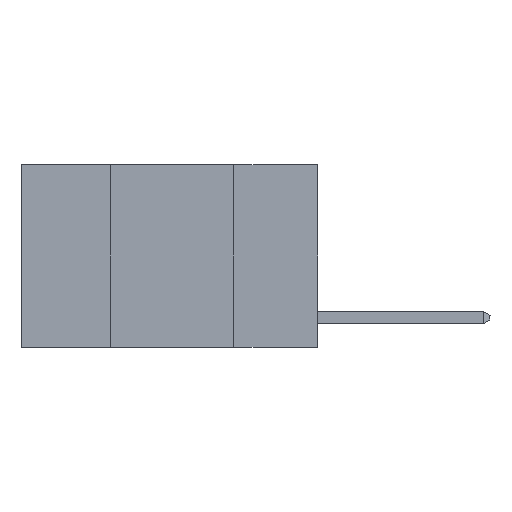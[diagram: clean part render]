
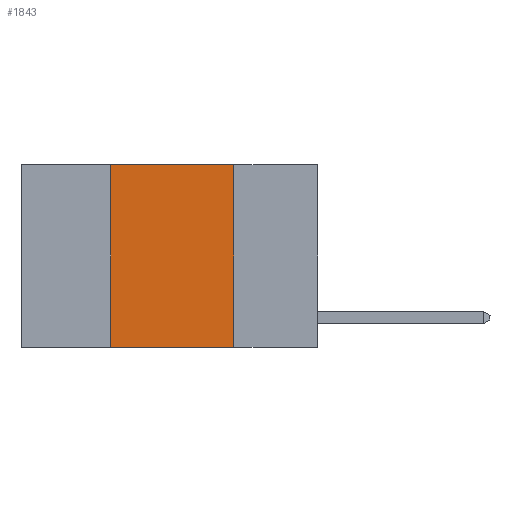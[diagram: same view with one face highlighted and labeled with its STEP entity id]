
A CAD part, left-side view. The second image highlights one B-rep face of the part: STEP entity #1843.
In plain terms, the highlighted planar face has unit normal (-1, 0, 0).
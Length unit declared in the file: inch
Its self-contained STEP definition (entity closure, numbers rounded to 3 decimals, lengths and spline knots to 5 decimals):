
#255 = EDGE_CURVE ( 'NONE', #11716, #3188, #11591, .T. ) ;
#520 = DIRECTION ( 'NONE',  ( 0., 0., -1. ) ) ;
#623 = LINE ( 'NONE', #10153, #10955 ) ;
#773 = EDGE_CURVE ( 'NONE', #4697, #6847, #623, .T. ) ;
#774 = AXIS2_PLACEMENT_3D ( 'NONE', #5759, #6787, #520 ) ;
#1813 = ORIENTED_EDGE ( 'NONE', *, *, #255, .T. ) ;
#1843 = ADVANCED_FACE ( 'NONE', ( #6644 ), #11828, .F. ) ;
#1957 = CARTESIAN_POINT ( 'NONE',  ( 0., 0.42, -0.37 ) ) ;
#2440 = ORIENTED_EDGE ( 'NONE', *, *, #3088, .F. ) ;
#2998 = DIRECTION ( 'NONE',  ( 0., -1., 0. ) ) ;
#3088 = EDGE_CURVE ( 'NONE', #11716, #4697, #7552, .T. ) ;
#3188 = VERTEX_POINT ( 'NONE', #8435 ) ;
#3421 = VECTOR ( 'NONE', #2998, 39.37008 ) ;
#3844 = CARTESIAN_POINT ( 'NONE',  ( 0., 0.42, 0. ) ) ;
#4002 = DIRECTION ( 'NONE',  ( 0., -1., 0. ) ) ;
#4008 = EDGE_LOOP ( 'NONE', ( #4565, #5241, #2440, #1813 ) ) ;
#4195 = VECTOR ( 'NONE', #5495, 39.37008 ) ;
#4565 = ORIENTED_EDGE ( 'NONE', *, *, #7956, .F. ) ;
#4697 = VERTEX_POINT ( 'NONE', #3844 ) ;
#4828 = VECTOR ( 'NONE', #10329, 39.37008 ) ;
#4864 = LINE ( 'NONE', #8536, #4195 ) ;
#5241 = ORIENTED_EDGE ( 'NONE', *, *, #773, .F. ) ;
#5495 = DIRECTION ( 'NONE',  ( 0., 0., -1. ) ) ;
#5759 = CARTESIAN_POINT ( 'NONE',  ( 0., 0.6, 0. ) ) ;
#6644 = FACE_OUTER_BOUND ( 'NONE', #4008, .T. ) ;
#6787 = DIRECTION ( 'NONE',  ( 1., 0., 0. ) ) ;
#6847 = VERTEX_POINT ( 'NONE', #7661 ) ;
#7552 = LINE ( 'NONE', #11337, #4828 ) ;
#7661 = CARTESIAN_POINT ( 'NONE',  ( 0., 0.17, 0. ) ) ;
#7956 = EDGE_CURVE ( 'NONE', #6847, #3188, #4864, .T. ) ;
#8435 = CARTESIAN_POINT ( 'NONE',  ( 0., 0.17, -0.37 ) ) ;
#8536 = CARTESIAN_POINT ( 'NONE',  ( 0., 0.17, 0. ) ) ;
#10153 = CARTESIAN_POINT ( 'NONE',  ( 0., 0.6, 0. ) ) ;
#10206 = CARTESIAN_POINT ( 'NONE',  ( 0., 0.6, -0.37 ) ) ;
#10329 = DIRECTION ( 'NONE',  ( 0., 0., 1. ) ) ;
#10955 = VECTOR ( 'NONE', #4002, 39.37008 ) ;
#11337 = CARTESIAN_POINT ( 'NONE',  ( 0., 0.42, 0. ) ) ;
#11591 = LINE ( 'NONE', #10206, #3421 ) ;
#11716 = VERTEX_POINT ( 'NONE', #1957 ) ;
#11828 = PLANE ( 'NONE',  #774 ) ;
